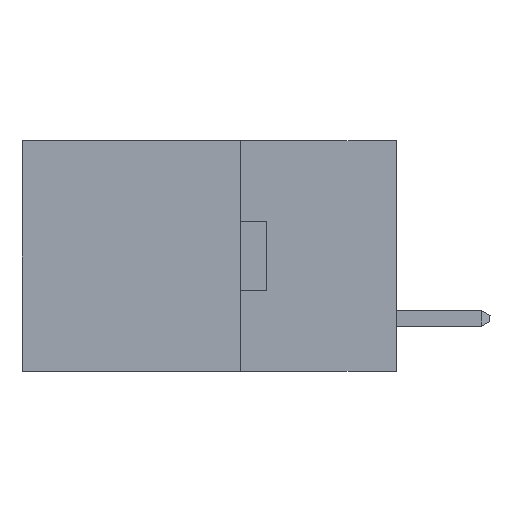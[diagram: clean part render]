
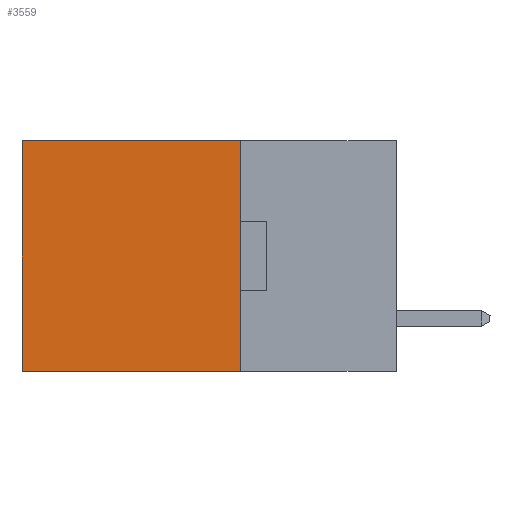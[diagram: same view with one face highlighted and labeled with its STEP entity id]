
A CAD part, left-side view. The second image highlights one B-rep face of the part: STEP entity #3559.
In plain terms, the highlighted planar face has unit normal (-1, 0, 0).
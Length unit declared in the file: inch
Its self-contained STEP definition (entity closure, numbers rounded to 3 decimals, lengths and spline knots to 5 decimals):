
#1609 = CARTESIAN_POINT ( 'NONE',  ( 0.2615, 0.25, 0. ) ) ;
#1717 = LINE ( 'NONE', #5820, #17380 ) ;
#2308 = DIRECTION ( 'NONE',  ( 0., 0., -1. ) ) ;
#3559 = ADVANCED_FACE ( 'NONE', ( #8992 ), #23668, .F. ) ;
#4740 = LINE ( 'NONE', #19607, #9669 ) ;
#4995 = DIRECTION ( 'NONE',  ( 1., 0., 0. ) ) ;
#5820 = CARTESIAN_POINT ( 'NONE',  ( 0.2615, 0.25, 0. ) ) ;
#6514 = ORIENTED_EDGE ( 'NONE', *, *, #8258, .T. ) ;
#7027 = CARTESIAN_POINT ( 'NONE',  ( 0.2615, 0.6, -0.37 ) ) ;
#8258 = EDGE_CURVE ( 'NONE', #17114, #17038, #1717, .T. ) ;
#8992 = FACE_OUTER_BOUND ( 'NONE', #19772, .T. ) ;
#9218 = ORIENTED_EDGE ( 'NONE', *, *, #22611, .F. ) ;
#9669 = VECTOR ( 'NONE', #15264, 39.37008 ) ;
#10553 = LINE ( 'NONE', #20473, #17228 ) ;
#12640 = EDGE_CURVE ( 'NONE', #24811, #22074, #10553, .T. ) ;
#12946 = CARTESIAN_POINT ( 'NONE',  ( 0.2615, 0.25, -0.37 ) ) ;
#13196 = CARTESIAN_POINT ( 'NONE',  ( 0.2615, 0.25, -0.37 ) ) ;
#13381 = DIRECTION ( 'NONE',  ( 0., 0., -1. ) ) ;
#13588 = ORIENTED_EDGE ( 'NONE', *, *, #12640, .F. ) ;
#15264 = DIRECTION ( 'NONE',  ( 0., 0., -1. ) ) ;
#16286 = EDGE_CURVE ( 'NONE', #17038, #22074, #4740, .T. ) ;
#17038 = VERTEX_POINT ( 'NONE', #21848 ) ;
#17088 = ORIENTED_EDGE ( 'NONE', *, *, #16286, .T. ) ;
#17114 = VERTEX_POINT ( 'NONE', #1609 ) ;
#17228 = VECTOR ( 'NONE', #22490, 39.37008 ) ;
#17380 = VECTOR ( 'NONE', #26647, 39.37008 ) ;
#19359 = CARTESIAN_POINT ( 'NONE',  ( 0.2615, 0.25, -0.37 ) ) ;
#19607 = CARTESIAN_POINT ( 'NONE',  ( 0.2615, 0.6, -0.37 ) ) ;
#19772 = EDGE_LOOP ( 'NONE', ( #17088, #13588, #9218, #6514 ) ) ;
#20473 = CARTESIAN_POINT ( 'NONE',  ( 0.2615, 0.25, -0.37 ) ) ;
#20979 = LINE ( 'NONE', #19359, #22819 ) ;
#21848 = CARTESIAN_POINT ( 'NONE',  ( 0.2615, 0.6, 0. ) ) ;
#22074 = VERTEX_POINT ( 'NONE', #7027 ) ;
#22490 = DIRECTION ( 'NONE',  ( 0., 1., 0. ) ) ;
#22611 = EDGE_CURVE ( 'NONE', #17114, #24811, #20979, .T. ) ;
#22819 = VECTOR ( 'NONE', #2308, 39.37008 ) ;
#23668 = PLANE ( 'NONE',  #24235 ) ;
#24235 = AXIS2_PLACEMENT_3D ( 'NONE', #12946, #4995, #13381 ) ;
#24811 = VERTEX_POINT ( 'NONE', #13196 ) ;
#26647 = DIRECTION ( 'NONE',  ( 0., 1., 0. ) ) ;
